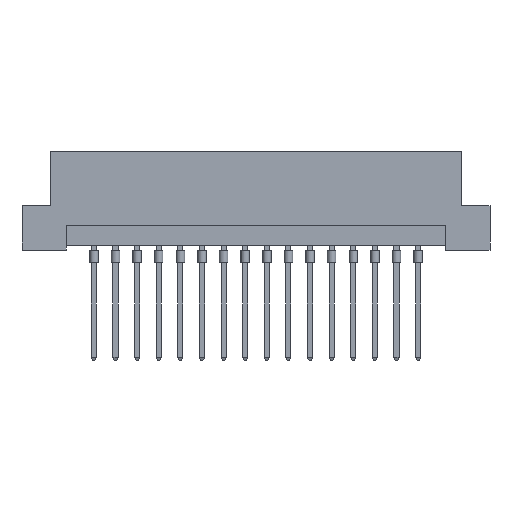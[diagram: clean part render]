
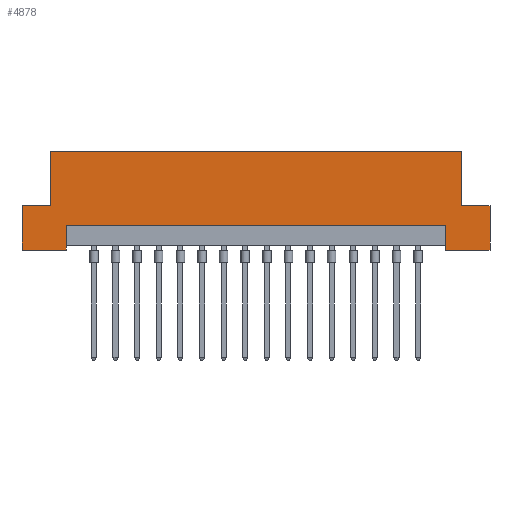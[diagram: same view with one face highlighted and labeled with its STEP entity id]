
A CAD part, front view. The second image highlights one B-rep face of the part: STEP entity #4878.
In plain terms, the highlighted planar face has unit normal (0, -1, 0).
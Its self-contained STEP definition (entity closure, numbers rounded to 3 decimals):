
#2 = LINE ( 'NONE', #197, #4168 ) ;
#12 = VECTOR ( 'NONE', #1180, 1000. ) ;
#44 = DIRECTION ( 'NONE',  ( 0., 0., 1. ) ) ;
#119 = LINE ( 'NONE', #3219, #1379 ) ;
#194 = VERTEX_POINT ( 'NONE', #7258 ) ;
#197 = CARTESIAN_POINT ( 'NONE',  ( -24.2, 0., 5.2 ) ) ;
#491 = CARTESIAN_POINT ( 'NONE',  ( 24.2, 0., 5.2 ) ) ;
#669 = EDGE_CURVE ( 'NONE', #4853, #3060, #2, .T. ) ;
#674 = CARTESIAN_POINT ( 'NONE',  ( 24.2, 0., 11.6 ) ) ;
#698 = CARTESIAN_POINT ( 'NONE',  ( 22.3, 0., 2.9 ) ) ;
#944 = EDGE_CURVE ( 'NONE', #4578, #5245, #6729, .T. ) ;
#1180 = DIRECTION ( 'NONE',  ( -1., 0., 0. ) ) ;
#1251 = CARTESIAN_POINT ( 'NONE',  ( -27.5, 0., 11.6 ) ) ;
#1379 = VECTOR ( 'NONE', #9441, 1000. ) ;
#1383 = CARTESIAN_POINT ( 'NONE',  ( 27.5, 0., 5.2 ) ) ;
#1457 = CARTESIAN_POINT ( 'NONE',  ( -24.2, 0., 5.2 ) ) ;
#1514 = LINE ( 'NONE', #7649, #7229 ) ;
#1731 = VECTOR ( 'NONE', #9936, 1000. ) ;
#1913 = CARTESIAN_POINT ( 'NONE',  ( 22.3, 0., 0.5 ) ) ;
#1943 = EDGE_CURVE ( 'NONE', #3060, #2695, #9142, .T. ) ;
#2419 = VECTOR ( 'NONE', #8424, 1000. ) ;
#2515 = ORIENTED_EDGE ( 'NONE', *, *, #6214, .F. ) ;
#2606 = CARTESIAN_POINT ( 'NONE',  ( 22.3, 0., 2.9 ) ) ;
#2695 = VERTEX_POINT ( 'NONE', #674 ) ;
#3060 = VERTEX_POINT ( 'NONE', #4534 ) ;
#3219 = CARTESIAN_POINT ( 'NONE',  ( -27.5, 0., 0. ) ) ;
#3759 = CARTESIAN_POINT ( 'NONE',  ( 27.5, 0., 0. ) ) ;
#3797 = CARTESIAN_POINT ( 'NONE',  ( -27.5, 0., 11.6 ) ) ;
#3874 = EDGE_CURVE ( 'NONE', #4578, #194, #7436, .T. ) ;
#4106 = DIRECTION ( 'NONE',  ( 0., 1., 0. ) ) ;
#4146 = EDGE_LOOP ( 'NONE', ( #4547, #8556, #7910, #2515, #9669, #9793, #6168, #4631, #6885, #9335, #6449, #5384 ) ) ;
#4168 = VECTOR ( 'NONE', #9379, 1000. ) ;
#4292 = CARTESIAN_POINT ( 'NONE',  ( -27.5, 0., 0. ) ) ;
#4330 = LINE ( 'NONE', #7499, #8004 ) ;
#4416 = AXIS2_PLACEMENT_3D ( 'NONE', #3797, #4106, #6457 ) ;
#4534 = CARTESIAN_POINT ( 'NONE',  ( -24.2, 0., 11.6 ) ) ;
#4547 = ORIENTED_EDGE ( 'NONE', *, *, #944, .F. ) ;
#4572 = FACE_OUTER_BOUND ( 'NONE', #4146, .T. ) ;
#4578 = VERTEX_POINT ( 'NONE', #2606 ) ;
#4625 = PLANE ( 'NONE',  #4416 ) ;
#4631 = ORIENTED_EDGE ( 'NONE', *, *, #669, .F. ) ;
#4853 = VERTEX_POINT ( 'NONE', #1457 ) ;
#4878 = ADVANCED_FACE ( 'NONE', ( #4572 ), #4625, .F. ) ;
#4920 = VERTEX_POINT ( 'NONE', #9503 ) ;
#4943 = VECTOR ( 'NONE', #6862, 1000. ) ;
#5061 = DIRECTION ( 'NONE',  ( 1., 0., 0. ) ) ;
#5245 = VERTEX_POINT ( 'NONE', #6815 ) ;
#5384 = ORIENTED_EDGE ( 'NONE', *, *, #8399, .F. ) ;
#5501 = EDGE_CURVE ( 'NONE', #8235, #5540, #119, .T. ) ;
#5540 = VERTEX_POINT ( 'NONE', #4292 ) ;
#5604 = CARTESIAN_POINT ( 'NONE',  ( -27.5, 0., 5.2 ) ) ;
#5714 = CARTESIAN_POINT ( 'NONE',  ( -27.5, 0., 0. ) ) ;
#6080 = CARTESIAN_POINT ( 'NONE',  ( 27.5, 0., 5.2 ) ) ;
#6120 = DIRECTION ( 'NONE',  ( 1., 0., 0. ) ) ;
#6168 = ORIENTED_EDGE ( 'NONE', *, *, #1943, .F. ) ;
#6214 = EDGE_CURVE ( 'NONE', #7522, #4920, #9794, .T. ) ;
#6228 = EDGE_CURVE ( 'NONE', #5540, #8287, #6682, .T. ) ;
#6449 = ORIENTED_EDGE ( 'NONE', *, *, #5501, .F. ) ;
#6457 = DIRECTION ( 'NONE',  ( 0., 0., 1. ) ) ;
#6472 = CARTESIAN_POINT ( 'NONE',  ( -22.3, 0., 0. ) ) ;
#6574 = DIRECTION ( 'NONE',  ( 0., 0., -1. ) ) ;
#6608 = LINE ( 'NONE', #7322, #7871 ) ;
#6682 = LINE ( 'NONE', #7506, #7484 ) ;
#6683 = VECTOR ( 'NONE', #7276, 1000. ) ;
#6729 = LINE ( 'NONE', #698, #1731 ) ;
#6815 = CARTESIAN_POINT ( 'NONE',  ( -22.3, 0., 2.9 ) ) ;
#6862 = DIRECTION ( 'NONE',  ( 1., 0., 0. ) ) ;
#6885 = ORIENTED_EDGE ( 'NONE', *, *, #8767, .F. ) ;
#7017 = VERTEX_POINT ( 'NONE', #491 ) ;
#7229 = VECTOR ( 'NONE', #44, 1000. ) ;
#7258 = CARTESIAN_POINT ( 'NONE',  ( 22.3, 0., 0. ) ) ;
#7276 = DIRECTION ( 'NONE',  ( 0., 0., -1. ) ) ;
#7322 = CARTESIAN_POINT ( 'NONE',  ( -27.5, 0., 5.2 ) ) ;
#7436 = LINE ( 'NONE', #1913, #6683 ) ;
#7484 = VECTOR ( 'NONE', #8267, 1000. ) ;
#7499 = CARTESIAN_POINT ( 'NONE',  ( -22.3, 0., 0.5 ) ) ;
#7506 = CARTESIAN_POINT ( 'NONE',  ( -27.5, 0., 0. ) ) ;
#7522 = VERTEX_POINT ( 'NONE', #6080 ) ;
#7649 = CARTESIAN_POINT ( 'NONE',  ( 24.2, 0., 5.2 ) ) ;
#7708 = VECTOR ( 'NONE', #6120, 1000. ) ;
#7871 = VECTOR ( 'NONE', #5061, 1000. ) ;
#7910 = ORIENTED_EDGE ( 'NONE', *, *, #9215, .F. ) ;
#8004 = VECTOR ( 'NONE', #6574, 1000. ) ;
#8175 = LINE ( 'NONE', #5714, #12 ) ;
#8235 = VERTEX_POINT ( 'NONE', #6472 ) ;
#8267 = DIRECTION ( 'NONE',  ( 0., 0., 1. ) ) ;
#8287 = VERTEX_POINT ( 'NONE', #5604 ) ;
#8377 = LINE ( 'NONE', #1383, #7708 ) ;
#8399 = EDGE_CURVE ( 'NONE', #5245, #8235, #4330, .T. ) ;
#8424 = DIRECTION ( 'NONE',  ( 0., 0., -1. ) ) ;
#8556 = ORIENTED_EDGE ( 'NONE', *, *, #3874, .T. ) ;
#8767 = EDGE_CURVE ( 'NONE', #8287, #4853, #6608, .T. ) ;
#9142 = LINE ( 'NONE', #1251, #4943 ) ;
#9215 = EDGE_CURVE ( 'NONE', #4920, #194, #8175, .T. ) ;
#9335 = ORIENTED_EDGE ( 'NONE', *, *, #6228, .F. ) ;
#9379 = DIRECTION ( 'NONE',  ( 0., 0., 1. ) ) ;
#9416 = EDGE_CURVE ( 'NONE', #7017, #7522, #8377, .T. ) ;
#9441 = DIRECTION ( 'NONE',  ( -1., 0., 0. ) ) ;
#9503 = CARTESIAN_POINT ( 'NONE',  ( 27.5, 0., 0. ) ) ;
#9669 = ORIENTED_EDGE ( 'NONE', *, *, #9416, .F. ) ;
#9793 = ORIENTED_EDGE ( 'NONE', *, *, #10047, .T. ) ;
#9794 = LINE ( 'NONE', #3759, #2419 ) ;
#9936 = DIRECTION ( 'NONE',  ( -1., 0., 0. ) ) ;
#10047 = EDGE_CURVE ( 'NONE', #7017, #2695, #1514, .T. ) ;
